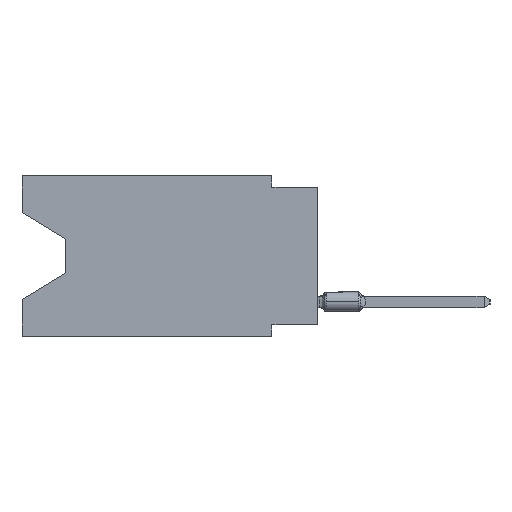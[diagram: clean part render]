
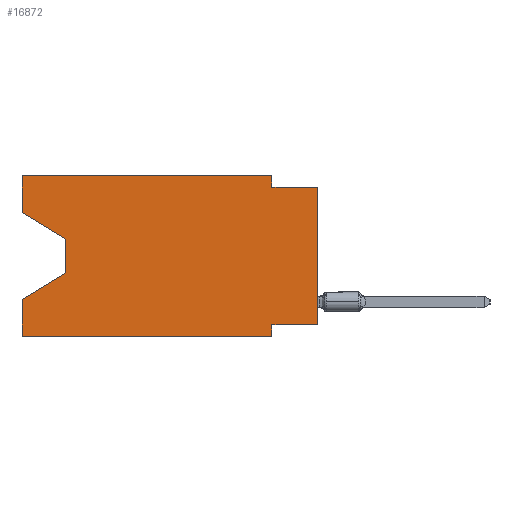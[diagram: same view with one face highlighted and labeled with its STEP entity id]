
A CAD part, left-side view. The second image highlights one B-rep face of the part: STEP entity #16872.
In plain terms, the highlighted planar face has unit normal (-1, 0, 0).
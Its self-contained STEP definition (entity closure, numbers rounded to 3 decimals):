
#150 = EDGE_CURVE ( 'NONE', #3417, #10435, #27973, .T. ) ;
#893 = VECTOR ( 'NONE', #22048, 1000. ) ;
#1729 = LINE ( 'NONE', #25341, #893 ) ;
#1985 = CARTESIAN_POINT ( 'NONE',  ( 0., 13.97, -3.505 ) ) ;
#3067 = VECTOR ( 'NONE', #19084, 1000. ) ;
#3417 = VERTEX_POINT ( 'NONE', #18289 ) ;
#3527 = VECTOR ( 'NONE', #16145, 1000. ) ;
#4184 = LINE ( 'NONE', #21606, #3067 ) ;
#4231 = CARTESIAN_POINT ( 'NONE',  ( 0., 16.383, 0. ) ) ;
#4337 = CARTESIAN_POINT ( 'NONE',  ( 0., 2.54, -8.89 ) ) ;
#4336 = CARTESIAN_POINT ( 'NONE',  ( 0., 0., -0.635 ) ) ;
#5528 = CARTESIAN_POINT ( 'NONE',  ( 0., 16.383, 0. ) ) ;
#6192 = CARTESIAN_POINT ( 'NONE',  ( 0., 2.54, -0.635 ) ) ;
#6428 = VERTEX_POINT ( 'NONE', #31929 ) ;
#7056 = DIRECTION ( 'NONE',  ( 0., 0., -1. ) ) ;
#7435 = LINE ( 'NONE', #4337, #15298 ) ;
#7755 = DIRECTION ( 'NONE',  ( 0., 0.855, -0.519 ) ) ;
#8043 = ORIENTED_EDGE ( 'NONE', *, *, #10554, .T. ) ;
#8840 = VECTOR ( 'NONE', #34456, 1000. ) ;
#9140 = ORIENTED_EDGE ( 'NONE', *, *, #26238, .F. ) ;
#9426 = VERTEX_POINT ( 'NONE', #14686 ) ;
#9949 = LINE ( 'NONE', #33525, #27049 ) ;
#10105 = DIRECTION ( 'NONE',  ( 0., 0., 1. ) ) ;
#10296 = CARTESIAN_POINT ( 'NONE',  ( 0., 16.383, -8.89 ) ) ;
#10410 = DIRECTION ( 'NONE',  ( 0., 0., 1. ) ) ;
#10435 = VERTEX_POINT ( 'NONE', #33509 ) ;
#10451 = LINE ( 'NONE', #37504, #22593 ) ;
#10554 = EDGE_CURVE ( 'NONE', #30501, #28619, #10879, .T. ) ;
#10879 = LINE ( 'NONE', #1985, #8840 ) ;
#11518 = DIRECTION ( 'NONE',  ( 1., 0., 0. ) ) ;
#11864 = ORIENTED_EDGE ( 'NONE', *, *, #29642, .T. ) ;
#12757 = ORIENTED_EDGE ( 'NONE', *, *, #16031, .F. ) ;
#12938 = VERTEX_POINT ( 'NONE', #34700 ) ;
#13693 = ORIENTED_EDGE ( 'NONE', *, *, #16974, .F. ) ;
#13875 = ORIENTED_EDGE ( 'NONE', *, *, #28924, .F. ) ;
#14686 = CARTESIAN_POINT ( 'NONE',  ( 0., 0., -8.255 ) ) ;
#15265 = EDGE_CURVE ( 'NONE', #31586, #12938, #36892, .T. ) ;
#15298 = VECTOR ( 'NONE', #15949, 1000. ) ;
#15949 = DIRECTION ( 'NONE',  ( 0., 0., -1. ) ) ;
#16031 = EDGE_CURVE ( 'NONE', #21177, #24743, #7435, .T. ) ;
#16145 = DIRECTION ( 'NONE',  ( 0., -1., 0. ) ) ;
#16872 = ADVANCED_FACE ( 'NONE', ( #38004 ), #34899, .F. ) ;
#16974 = EDGE_CURVE ( 'NONE', #10435, #17264, #9949, .T. ) ;
#17074 = CARTESIAN_POINT ( 'NONE',  ( 0., 13.97, -3.505 ) ) ;
#17264 = VERTEX_POINT ( 'NONE', #6192 ) ;
#18289 = CARTESIAN_POINT ( 'NONE',  ( 0., 16.383, 0. ) ) ;
#18489 = EDGE_CURVE ( 'NONE', #19310, #30501, #4184, .T. ) ;
#18988 = VECTOR ( 'NONE', #22951, 1000. ) ;
#19084 = DIRECTION ( 'NONE',  ( 0., -0.855, -0.519 ) ) ;
#19146 = CARTESIAN_POINT ( 'NONE',  ( 0., 16.383, -8.89 ) ) ;
#19310 = VERTEX_POINT ( 'NONE', #21280 ) ;
#19867 = CARTESIAN_POINT ( 'NONE',  ( 0., 0., -8.255 ) ) ;
#19926 = ORIENTED_EDGE ( 'NONE', *, *, #34504, .F. ) ;
#20795 = EDGE_LOOP ( 'NONE', ( #27056, #8043, #22976, #26824, #11864, #12757, #19926, #33530, #13875, #13693, #28000, #9140 ) ) ;
#21177 = VERTEX_POINT ( 'NONE', #22854 ) ;
#21280 = CARTESIAN_POINT ( 'NONE',  ( 0., 16.383, -2.038 ) ) ;
#21606 = CARTESIAN_POINT ( 'NONE',  ( 0., 16.383, -2.038 ) ) ;
#22039 = DIRECTION ( 'NONE',  ( 0., -1., 0. ) ) ;
#22048 = DIRECTION ( 'NONE',  ( 0., 0., 1. ) ) ;
#22593 = VECTOR ( 'NONE', #7755, 1000. ) ;
#22647 = VECTOR ( 'NONE', #31846, 1000. ) ;
#22770 = LINE ( 'NONE', #19867, #22647 ) ;
#22854 = CARTESIAN_POINT ( 'NONE',  ( 0., 2.54, -8.255 ) ) ;
#22951 = DIRECTION ( 'NONE',  ( 0., -1., 0. ) ) ;
#22976 = ORIENTED_EDGE ( 'NONE', *, *, #33182, .T. ) ;
#23234 = CARTESIAN_POINT ( 'NONE',  ( 0., 2.54, -8.89 ) ) ;
#23324 = DIRECTION ( 'NONE',  ( 0., 0., -1. ) ) ;
#24743 = VERTEX_POINT ( 'NONE', #23234 ) ;
#25037 = LINE ( 'NONE', #4336, #3527 ) ;
#25341 = CARTESIAN_POINT ( 'NONE',  ( 0., 16.383, 0. ) ) ;
#25823 = VECTOR ( 'NONE', #10105, 1000. ) ;
#26238 = EDGE_CURVE ( 'NONE', #19310, #3417, #1729, .T. ) ;
#26824 = ORIENTED_EDGE ( 'NONE', *, *, #15265, .F. ) ;
#27049 = VECTOR ( 'NONE', #7056, 1000. ) ;
#27056 = ORIENTED_EDGE ( 'NONE', *, *, #18489, .T. ) ;
#27129 = LINE ( 'NONE', #36582, #25823 ) ;
#27973 = LINE ( 'NONE', #32208, #18988 ) ;
#28000 = ORIENTED_EDGE ( 'NONE', *, *, #150, .F. ) ;
#28619 = VERTEX_POINT ( 'NONE', #34376 ) ;
#28871 = VECTOR ( 'NONE', #10410, 1000. ) ;
#28924 = EDGE_CURVE ( 'NONE', #17264, #6428, #25037, .T. ) ;
#29642 = EDGE_CURVE ( 'NONE', #31586, #24743, #31124, .T. ) ;
#30369 = EDGE_CURVE ( 'NONE', #9426, #6428, #27129, .T. ) ;
#30501 = VERTEX_POINT ( 'NONE', #17074 ) ;
#31124 = LINE ( 'NONE', #19146, #36223 ) ;
#31586 = VERTEX_POINT ( 'NONE', #10296 ) ;
#31846 = DIRECTION ( 'NONE',  ( 0., 1., 0. ) ) ;
#31929 = CARTESIAN_POINT ( 'NONE',  ( 0., 0., -0.635 ) ) ;
#32208 = CARTESIAN_POINT ( 'NONE',  ( 0., 16.383, 0. ) ) ;
#33182 = EDGE_CURVE ( 'NONE', #28619, #12938, #10451, .T. ) ;
#33509 = CARTESIAN_POINT ( 'NONE',  ( 0., 2.54, 0. ) ) ;
#33525 = CARTESIAN_POINT ( 'NONE',  ( 0., 2.54, 0. ) ) ;
#33530 = ORIENTED_EDGE ( 'NONE', *, *, #30369, .T. ) ;
#34376 = CARTESIAN_POINT ( 'NONE',  ( 0., 13.97, -5.385 ) ) ;
#34456 = DIRECTION ( 'NONE',  ( 0., 0., -1. ) ) ;
#34504 = EDGE_CURVE ( 'NONE', #9426, #21177, #22770, .T. ) ;
#34700 = CARTESIAN_POINT ( 'NONE',  ( 0., 16.383, -6.852 ) ) ;
#34899 = PLANE ( 'NONE',  #36308 ) ;
#36223 = VECTOR ( 'NONE', #22039, 1000. ) ;
#36308 = AXIS2_PLACEMENT_3D ( 'NONE', #5528, #11518, #23324 ) ;
#36582 = CARTESIAN_POINT ( 'NONE',  ( 0., 0., 0. ) ) ;
#36892 = LINE ( 'NONE', #4231, #28871 ) ;
#37504 = CARTESIAN_POINT ( 'NONE',  ( 0., 13.97, -5.385 ) ) ;
#38004 = FACE_OUTER_BOUND ( 'NONE', #20795, .T. ) ;
